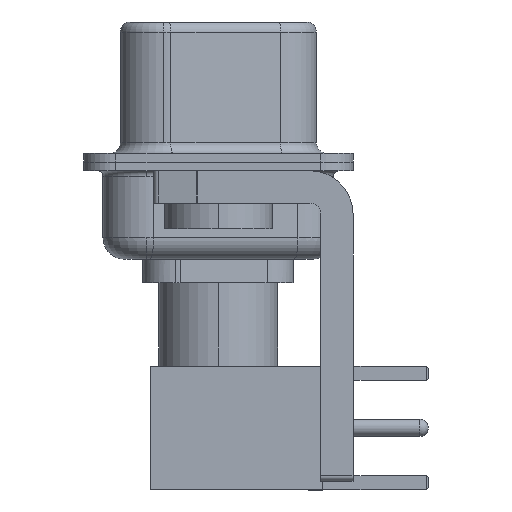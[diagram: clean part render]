
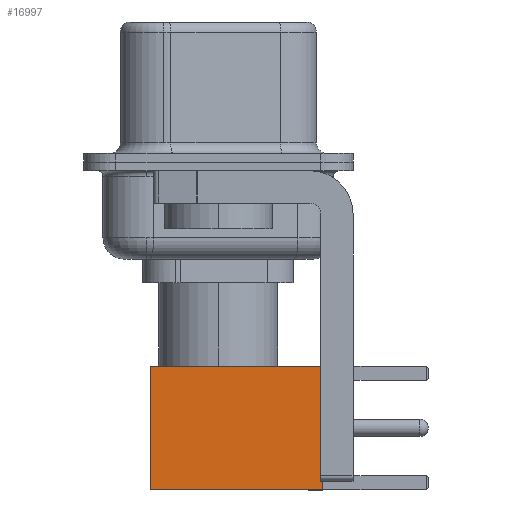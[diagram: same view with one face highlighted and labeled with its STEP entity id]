
A CAD part, left-side view. The second image highlights one B-rep face of the part: STEP entity #16997.
In plain terms, the highlighted face is planar.
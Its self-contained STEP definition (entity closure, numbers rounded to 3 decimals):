
#177 = DIRECTION ( 'NONE',  ( -1., 0., 0. ) ) ;
#474 = VECTOR ( 'NONE', #14438, 1000. ) ;
#1837 = VERTEX_POINT ( 'NONE', #19209 ) ;
#2130 = EDGE_CURVE ( 'NONE', #18148, #14500, #2921, .T. ) ;
#2492 = DIRECTION ( 'NONE',  ( 0., 0., 1. ) ) ;
#2537 = CARTESIAN_POINT ( 'NONE',  ( 2.875, 2.875, 0. ) ) ;
#2921 = LINE ( 'NONE', #7282, #19392 ) ;
#2969 = LINE ( 'NONE', #4944, #16894 ) ;
#4230 = VECTOR ( 'NONE', #8472, 1000. ) ;
#4252 = PLANE ( 'NONE',  #5190 ) ;
#4619 = EDGE_LOOP ( 'NONE', ( #11455, #12914, #5719, #5879 ) ) ;
#4944 = CARTESIAN_POINT ( 'NONE',  ( 0., 2.875, 0. ) ) ;
#5029 = CARTESIAN_POINT ( 'NONE',  ( 2.875, 2.875, 8. ) ) ;
#5190 = AXIS2_PLACEMENT_3D ( 'NONE', #8932, #10716, #2492 ) ;
#5719 = ORIENTED_EDGE ( 'NONE', *, *, #7279, .F. ) ;
#5879 = ORIENTED_EDGE ( 'NONE', *, *, #2130, .F. ) ;
#7115 = EDGE_CURVE ( 'NONE', #17908, #1837, #2969, .T. ) ;
#7279 = EDGE_CURVE ( 'NONE', #14500, #1837, #16206, .T. ) ;
#7282 = CARTESIAN_POINT ( 'NONE',  ( 0., 2.875, 8. ) ) ;
#8163 = CARTESIAN_POINT ( 'NONE',  ( -2.875, 2.875, 8. ) ) ;
#8472 = DIRECTION ( 'NONE',  ( 0., 0., -1. ) ) ;
#8932 = CARTESIAN_POINT ( 'NONE',  ( 2.875, 2.875, 0. ) ) ;
#10428 = DIRECTION ( 'NONE',  ( -1., 0., 0. ) ) ;
#10716 = DIRECTION ( 'NONE',  ( 0., 1., 0. ) ) ;
#11455 = ORIENTED_EDGE ( 'NONE', *, *, #14443, .T. ) ;
#12914 = ORIENTED_EDGE ( 'NONE', *, *, #7115, .T. ) ;
#13375 = CARTESIAN_POINT ( 'NONE',  ( -2.875, 2.875, 0. ) ) ;
#14438 = DIRECTION ( 'NONE',  ( 0., 0., -1. ) ) ;
#14443 = EDGE_CURVE ( 'NONE', #18148, #17908, #19232, .T. ) ;
#14500 = VERTEX_POINT ( 'NONE', #8163 ) ;
#16206 = LINE ( 'NONE', #13375, #4230 ) ;
#16790 = FACE_OUTER_BOUND ( 'NONE', #4619, .T. ) ;
#16894 = VECTOR ( 'NONE', #177, 1000. ) ;
#16997 = ADVANCED_FACE ( 'NONE', ( #16790 ), #4252, .T. ) ;
#17908 = VERTEX_POINT ( 'NONE', #2537 ) ;
#18148 = VERTEX_POINT ( 'NONE', #5029 ) ;
#18923 = CARTESIAN_POINT ( 'NONE',  ( 2.875, 2.875, 0. ) ) ;
#19209 = CARTESIAN_POINT ( 'NONE',  ( -2.875, 2.875, 0. ) ) ;
#19232 = LINE ( 'NONE', #18923, #474 ) ;
#19392 = VECTOR ( 'NONE', #10428, 1000. ) ;
